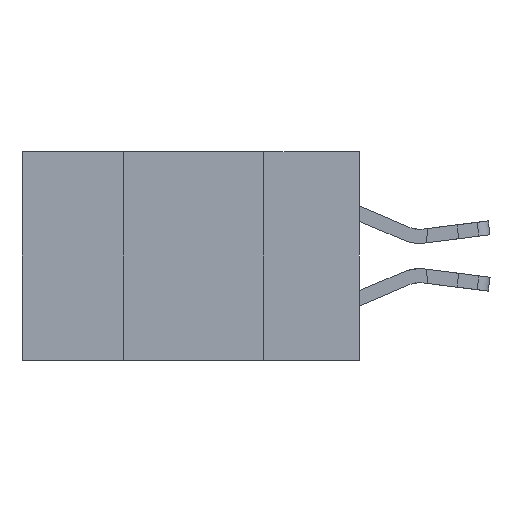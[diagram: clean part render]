
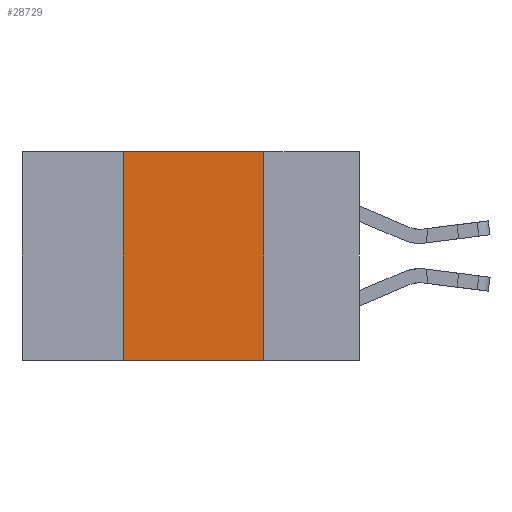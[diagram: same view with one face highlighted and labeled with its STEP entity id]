
A CAD part, left-side view. The second image highlights one B-rep face of the part: STEP entity #28729.
In plain terms, the highlighted planar face has unit normal (-1, 0, 0).
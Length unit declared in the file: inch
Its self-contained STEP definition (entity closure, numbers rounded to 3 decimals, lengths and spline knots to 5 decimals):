
#1168 = EDGE_CURVE ( 'NONE', #6297, #18601, #28783, .T. ) ;
#1188 = FACE_OUTER_BOUND ( 'NONE', #4002, .T. ) ;
#2220 = ORIENTED_EDGE ( 'NONE', *, *, #18403, .F. ) ;
#2747 = CARTESIAN_POINT ( 'NONE',  ( 0., 0.42, 0. ) ) ;
#2893 = DIRECTION ( 'NONE',  ( 0., 0., -1. ) ) ;
#3920 = CARTESIAN_POINT ( 'NONE',  ( 0., 0.6, -0.37 ) ) ;
#4002 = EDGE_LOOP ( 'NONE', ( #32747, #2220, #32153, #11159 ) ) ;
#4379 = DIRECTION ( 'NONE',  ( 0., -1., 0. ) ) ;
#5403 = PLANE ( 'NONE',  #11492 ) ;
#6297 = VERTEX_POINT ( 'NONE', #16859 ) ;
#7773 = CARTESIAN_POINT ( 'NONE',  ( 0., 0.6, 0. ) ) ;
#11159 = ORIENTED_EDGE ( 'NONE', *, *, #30317, .T. ) ;
#11492 = AXIS2_PLACEMENT_3D ( 'NONE', #7773, #28393, #12996 ) ;
#12352 = VECTOR ( 'NONE', #13322, 39.37008 ) ;
#12965 = CARTESIAN_POINT ( 'NONE',  ( 0., 0.17, 0. ) ) ;
#12996 = DIRECTION ( 'NONE',  ( 0., 0., -1. ) ) ;
#13322 = DIRECTION ( 'NONE',  ( 0., 0., 1. ) ) ;
#15996 = VECTOR ( 'NONE', #20342, 39.37008 ) ;
#16859 = CARTESIAN_POINT ( 'NONE',  ( 0., 0.42, -0.37 ) ) ;
#17010 = VECTOR ( 'NONE', #2893, 39.37008 ) ;
#18403 = EDGE_CURVE ( 'NONE', #18601, #22463, #32088, .T. ) ;
#18601 = VERTEX_POINT ( 'NONE', #2747 ) ;
#20342 = DIRECTION ( 'NONE',  ( 0., -1., 0. ) ) ;
#21691 = EDGE_CURVE ( 'NONE', #22463, #23781, #25509, .T. ) ;
#22463 = VERTEX_POINT ( 'NONE', #28990 ) ;
#23162 = CARTESIAN_POINT ( 'NONE',  ( 0., 0.6, 0. ) ) ;
#23781 = VERTEX_POINT ( 'NONE', #31666 ) ;
#25393 = CARTESIAN_POINT ( 'NONE',  ( 0., 0.42, 0. ) ) ;
#25509 = LINE ( 'NONE', #12965, #17010 ) ;
#26878 = LINE ( 'NONE', #3920, #32934 ) ;
#28393 = DIRECTION ( 'NONE',  ( 1., 0., 0. ) ) ;
#28729 = ADVANCED_FACE ( 'NONE', ( #1188 ), #5403, .F. ) ;
#28783 = LINE ( 'NONE', #25393, #12352 ) ;
#28990 = CARTESIAN_POINT ( 'NONE',  ( 0., 0.17, 0. ) ) ;
#30317 = EDGE_CURVE ( 'NONE', #6297, #23781, #26878, .T. ) ;
#31666 = CARTESIAN_POINT ( 'NONE',  ( 0., 0.17, -0.37 ) ) ;
#32088 = LINE ( 'NONE', #23162, #15996 ) ;
#32153 = ORIENTED_EDGE ( 'NONE', *, *, #1168, .F. ) ;
#32747 = ORIENTED_EDGE ( 'NONE', *, *, #21691, .F. ) ;
#32934 = VECTOR ( 'NONE', #4379, 39.37008 ) ;
